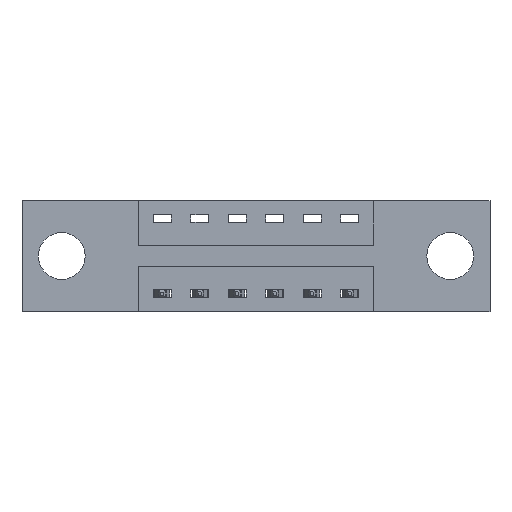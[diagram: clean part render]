
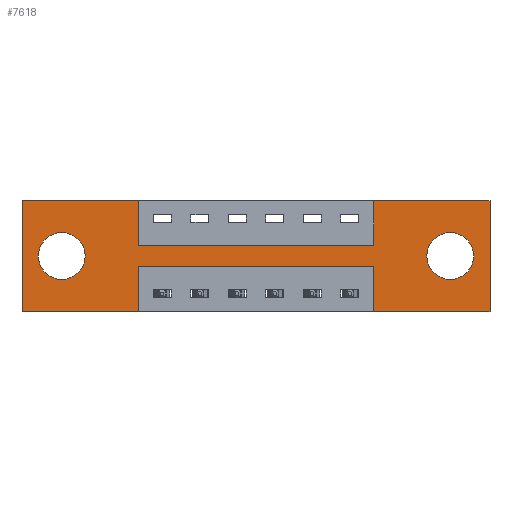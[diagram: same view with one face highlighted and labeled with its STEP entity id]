
A CAD part, front view. The second image highlights one B-rep face of the part: STEP entity #7618.
In plain terms, the highlighted planar face has unit normal (0, -1, 0).
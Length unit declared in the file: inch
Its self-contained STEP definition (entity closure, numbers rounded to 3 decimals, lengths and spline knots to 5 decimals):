
#19 = LINE ( 'NONE', #4729, #7029 ) ;
#31 = EDGE_CURVE ( 'NONE', #1222, #3871, #2668, .T. ) ;
#41 = EDGE_CURVE ( 'NONE', #6150, #8811, #3557, .T. ) ;
#191 = ORIENTED_EDGE ( 'NONE', *, *, #935, .F. ) ;
#284 = CARTESIAN_POINT ( 'NONE',  ( 0., 0., -0.37 ) ) ;
#324 = EDGE_LOOP ( 'NONE', ( #8713, #658 ) ) ;
#348 = VERTEX_POINT ( 'NONE', #2431 ) ;
#406 = VERTEX_POINT ( 'NONE', #1261 ) ;
#532 = ORIENTED_EDGE ( 'NONE', *, *, #1911, .F. ) ;
#552 = ORIENTED_EDGE ( 'NONE', *, *, #3383, .F. ) ;
#658 = ORIENTED_EDGE ( 'NONE', *, *, #31, .T. ) ;
#664 = AXIS2_PLACEMENT_3D ( 'NONE', #5314, #8726, #1868 ) ;
#686 = CARTESIAN_POINT ( 'NONE',  ( 1.56, 0., 0. ) ) ;
#779 = CARTESIAN_POINT ( 'NONE',  ( 1.4275, 0., -0.185 ) ) ;
#792 = CARTESIAN_POINT ( 'NONE',  ( 1.1725, 0., -0.15 ) ) ;
#813 = EDGE_CURVE ( 'NONE', #4842, #8606, #5442, .T. ) ;
#935 = EDGE_CURVE ( 'NONE', #3645, #406, #4186, .T. ) ;
#952 = CARTESIAN_POINT ( 'NONE',  ( 1.1725, 0., -0.22 ) ) ;
#1022 = VECTOR ( 'NONE', #6432, 39.37008 ) ;
#1129 = CARTESIAN_POINT ( 'NONE',  ( 0., 0., -0.37 ) ) ;
#1142 = CARTESIAN_POINT ( 'NONE',  ( 1.1725, 0., 0. ) ) ;
#1222 = VERTEX_POINT ( 'NONE', #2136 ) ;
#1261 = CARTESIAN_POINT ( 'NONE',  ( 0.3875, 0., -0.37 ) ) ;
#1308 = EDGE_CURVE ( 'NONE', #4043, #5974, #8132, .T. ) ;
#1379 = DIRECTION ( 'NONE',  ( 0., 1., 0. ) ) ;
#1538 = VECTOR ( 'NONE', #6727, 39.37008 ) ;
#1574 = CARTESIAN_POINT ( 'NONE',  ( 0.3875, 0., -0.37 ) ) ;
#1619 = FACE_BOUND ( 'NONE', #5233, .T. ) ;
#1675 = DIRECTION ( 'NONE',  ( 1., 0., 0. ) ) ;
#1731 = DIRECTION ( 'NONE',  ( 1., 0., 0. ) ) ;
#1779 = EDGE_CURVE ( 'NONE', #8750, #5520, #19, .T. ) ;
#1867 = LINE ( 'NONE', #3802, #4341 ) ;
#1868 = DIRECTION ( 'NONE',  ( 0., 0., 1. ) ) ;
#1892 = CIRCLE ( 'NONE', #3759, 0.078 ) ;
#1911 = EDGE_CURVE ( 'NONE', #406, #8750, #2595, .T. ) ;
#1976 = ORIENTED_EDGE ( 'NONE', *, *, #41, .F. ) ;
#2017 = CARTESIAN_POINT ( 'NONE',  ( 1.1725, 0., -0.37 ) ) ;
#2136 = CARTESIAN_POINT ( 'NONE',  ( 1.4275, 0., -0.263 ) ) ;
#2368 = CARTESIAN_POINT ( 'NONE',  ( 1.1725, 0., 0. ) ) ;
#2431 = CARTESIAN_POINT ( 'NONE',  ( 0.3875, 0., 0. ) ) ;
#2520 = ORIENTED_EDGE ( 'NONE', *, *, #3944, .T. ) ;
#2556 = ORIENTED_EDGE ( 'NONE', *, *, #7381, .F. ) ;
#2562 = LINE ( 'NONE', #5998, #3850 ) ;
#2589 = CARTESIAN_POINT ( 'NONE',  ( 1.1725, 0., -0.37 ) ) ;
#2595 = LINE ( 'NONE', #1129, #7175 ) ;
#2668 = CIRCLE ( 'NONE', #4567, 0.078 ) ;
#2761 = CARTESIAN_POINT ( 'NONE',  ( 0.1325, 0., -0.263 ) ) ;
#2827 = DIRECTION ( 'NONE',  ( 0., 0., 1. ) ) ;
#2875 = ORIENTED_EDGE ( 'NONE', *, *, #7199, .F. ) ;
#2883 = ORIENTED_EDGE ( 'NONE', *, *, #1308, .T. ) ;
#2938 = LINE ( 'NONE', #6285, #7248 ) ;
#3063 = AXIS2_PLACEMENT_3D ( 'NONE', #284, #4367, #6415 ) ;
#3383 = EDGE_CURVE ( 'NONE', #8606, #3645, #2562, .T. ) ;
#3446 = EDGE_CURVE ( 'NONE', #348, #5410, #4687, .T. ) ;
#3557 = LINE ( 'NONE', #686, #8343 ) ;
#3574 = CIRCLE ( 'NONE', #664, 0.078 ) ;
#3600 = EDGE_LOOP ( 'NONE', ( #191, #552, #8079, #8552, #1976, #7321, #2875, #2556, #3822, #4308, #6287, #532 ) ) ;
#3645 = VERTEX_POINT ( 'NONE', #4853 ) ;
#3665 = LINE ( 'NONE', #2368, #1022 ) ;
#3691 = DIRECTION ( 'NONE',  ( 1., 0., 0. ) ) ;
#3759 = AXIS2_PLACEMENT_3D ( 'NONE', #4370, #8411, #8866 ) ;
#3780 = FACE_OUTER_BOUND ( 'NONE', #3600, .T. ) ;
#3802 = CARTESIAN_POINT ( 'NONE',  ( 0.3875, 0., -0.15 ) ) ;
#3822 = ORIENTED_EDGE ( 'NONE', *, *, #3446, .F. ) ;
#3850 = VECTOR ( 'NONE', #8127, 39.37008 ) ;
#3871 = VERTEX_POINT ( 'NONE', #6668 ) ;
#3944 = EDGE_CURVE ( 'NONE', #5974, #4043, #3574, .T. ) ;
#3965 = CARTESIAN_POINT ( 'NONE',  ( 0., 0., -0.37 ) ) ;
#4007 = CARTESIAN_POINT ( 'NONE',  ( 1.56, 0., -0.37 ) ) ;
#4043 = VERTEX_POINT ( 'NONE', #2761 ) ;
#4186 = LINE ( 'NONE', #1574, #6419 ) ;
#4308 = ORIENTED_EDGE ( 'NONE', *, *, #4522, .F. ) ;
#4341 = VECTOR ( 'NONE', #1731, 39.37008 ) ;
#4367 = DIRECTION ( 'NONE',  ( 0., -1., 0. ) ) ;
#4370 = CARTESIAN_POINT ( 'NONE',  ( 1.4275, 0., -0.185 ) ) ;
#4520 = DIRECTION ( 'NONE',  ( 0., 0., 1. ) ) ;
#4522 = EDGE_CURVE ( 'NONE', #5520, #348, #2938, .T. ) ;
#4567 = AXIS2_PLACEMENT_3D ( 'NONE', #779, #1379, #6915 ) ;
#4569 = EDGE_CURVE ( 'NONE', #3871, #1222, #1892, .T. ) ;
#4581 = VECTOR ( 'NONE', #4794, 39.37008 ) ;
#4641 = VECTOR ( 'NONE', #1675, 39.37008 ) ;
#4642 = EDGE_CURVE ( 'NONE', #5165, #6150, #5120, .T. ) ;
#4687 = LINE ( 'NONE', #6639, #1538 ) ;
#4729 = CARTESIAN_POINT ( 'NONE',  ( 0., 0., 0. ) ) ;
#4794 = DIRECTION ( 'NONE',  ( 0., 0., 1. ) ) ;
#4842 = VERTEX_POINT ( 'NONE', #2017 ) ;
#4853 = CARTESIAN_POINT ( 'NONE',  ( 0.3875, 0., -0.22 ) ) ;
#5120 = LINE ( 'NONE', #7905, #4641 ) ;
#5127 = CARTESIAN_POINT ( 'NONE',  ( 0.1325, 0., -0.107 ) ) ;
#5165 = VERTEX_POINT ( 'NONE', #1142 ) ;
#5200 = PLANE ( 'NONE',  #3063 ) ;
#5233 = EDGE_LOOP ( 'NONE', ( #2520, #2883 ) ) ;
#5314 = CARTESIAN_POINT ( 'NONE',  ( 0.1325, 0., -0.185 ) ) ;
#5410 = VERTEX_POINT ( 'NONE', #8531 ) ;
#5442 = LINE ( 'NONE', #2589, #4581 ) ;
#5520 = VERTEX_POINT ( 'NONE', #5634 ) ;
#5634 = CARTESIAN_POINT ( 'NONE',  ( 0., 0., 0. ) ) ;
#5664 = EDGE_CURVE ( 'NONE', #8811, #4842, #7352, .T. ) ;
#5857 = VERTEX_POINT ( 'NONE', #792 ) ;
#5974 = VERTEX_POINT ( 'NONE', #5127 ) ;
#5998 = CARTESIAN_POINT ( 'NONE',  ( 0.3875, 0., -0.22 ) ) ;
#6021 = CARTESIAN_POINT ( 'NONE',  ( 1.56, 0., 0. ) ) ;
#6150 = VERTEX_POINT ( 'NONE', #6021 ) ;
#6155 = DIRECTION ( 'NONE',  ( -1., 0., 0. ) ) ;
#6278 = DIRECTION ( 'NONE',  ( 0., 0., -1. ) ) ;
#6285 = CARTESIAN_POINT ( 'NONE',  ( 0., 0., 0. ) ) ;
#6287 = ORIENTED_EDGE ( 'NONE', *, *, #1779, .F. ) ;
#6415 = DIRECTION ( 'NONE',  ( 0., 0., -1. ) ) ;
#6419 = VECTOR ( 'NONE', #6420, 39.37008 ) ;
#6420 = DIRECTION ( 'NONE',  ( 0., 0., -1. ) ) ;
#6432 = DIRECTION ( 'NONE',  ( 0., 0., 1. ) ) ;
#6633 = DIRECTION ( 'NONE',  ( -1., 0., 0. ) ) ;
#6639 = CARTESIAN_POINT ( 'NONE',  ( 0.3875, 0., 0. ) ) ;
#6668 = CARTESIAN_POINT ( 'NONE',  ( 1.4275, 0., -0.107 ) ) ;
#6727 = DIRECTION ( 'NONE',  ( 0., 0., -1. ) ) ;
#6915 = DIRECTION ( 'NONE',  ( 0., 0., -1. ) ) ;
#7029 = VECTOR ( 'NONE', #2827, 39.37008 ) ;
#7175 = VECTOR ( 'NONE', #6633, 39.37008 ) ;
#7192 = FACE_BOUND ( 'NONE', #324, .T. ) ;
#7199 = EDGE_CURVE ( 'NONE', #5857, #5165, #3665, .T. ) ;
#7248 = VECTOR ( 'NONE', #3691, 39.37008 ) ;
#7321 = ORIENTED_EDGE ( 'NONE', *, *, #4642, .F. ) ;
#7347 = DIRECTION ( 'NONE',  ( 0., 1., 0. ) ) ;
#7352 = LINE ( 'NONE', #3965, #7715 ) ;
#7381 = EDGE_CURVE ( 'NONE', #5410, #5857, #1867, .T. ) ;
#7573 = CARTESIAN_POINT ( 'NONE',  ( 0., 0., -0.37 ) ) ;
#7618 = ADVANCED_FACE ( 'NONE', ( #7192, #1619, #3780 ), #5200, .T. ) ;
#7715 = VECTOR ( 'NONE', #6155, 39.37008 ) ;
#7905 = CARTESIAN_POINT ( 'NONE',  ( 0., 0., 0. ) ) ;
#8079 = ORIENTED_EDGE ( 'NONE', *, *, #813, .F. ) ;
#8127 = DIRECTION ( 'NONE',  ( -1., 0., 0. ) ) ;
#8132 = CIRCLE ( 'NONE', #8419, 0.078 ) ;
#8343 = VECTOR ( 'NONE', #6278, 39.37008 ) ;
#8411 = DIRECTION ( 'NONE',  ( 0., 1., 0. ) ) ;
#8419 = AXIS2_PLACEMENT_3D ( 'NONE', #8469, #7347, #4520 ) ;
#8469 = CARTESIAN_POINT ( 'NONE',  ( 0.1325, 0., -0.185 ) ) ;
#8531 = CARTESIAN_POINT ( 'NONE',  ( 0.3875, 0., -0.15 ) ) ;
#8552 = ORIENTED_EDGE ( 'NONE', *, *, #5664, .F. ) ;
#8606 = VERTEX_POINT ( 'NONE', #952 ) ;
#8713 = ORIENTED_EDGE ( 'NONE', *, *, #4569, .T. ) ;
#8726 = DIRECTION ( 'NONE',  ( 0., 1., 0. ) ) ;
#8750 = VERTEX_POINT ( 'NONE', #7573 ) ;
#8811 = VERTEX_POINT ( 'NONE', #4007 ) ;
#8866 = DIRECTION ( 'NONE',  ( 0., 0., -1. ) ) ;
